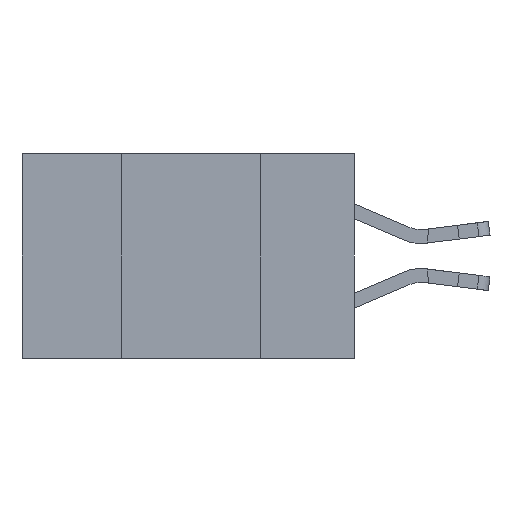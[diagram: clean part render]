
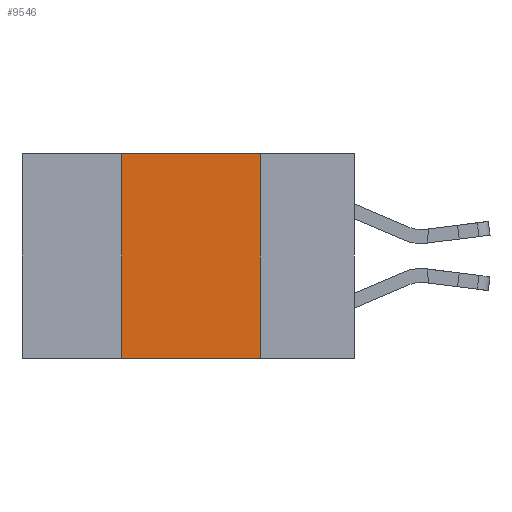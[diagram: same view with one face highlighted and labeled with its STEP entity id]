
A CAD part, left-side view. The second image highlights one B-rep face of the part: STEP entity #9546.
In plain terms, the highlighted planar face has unit normal (-1, 0, 0).
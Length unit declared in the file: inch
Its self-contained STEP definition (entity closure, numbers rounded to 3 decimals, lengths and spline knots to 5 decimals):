
#5 = ORIENTED_EDGE ( 'NONE', *, *, #11886, .F. ) ;
#1324 = CARTESIAN_POINT ( 'NONE',  ( 0., 0.6, 0. ) ) ;
#1542 = EDGE_CURVE ( 'NONE', #3734, #3479, #6570, .T. ) ;
#1946 = CARTESIAN_POINT ( 'NONE',  ( 0., 0.42, 0. ) ) ;
#2038 = VECTOR ( 'NONE', #15646, 39.37008 ) ;
#2591 = DIRECTION ( 'NONE',  ( 1., 0., 0. ) ) ;
#2919 = CARTESIAN_POINT ( 'NONE',  ( 0., 0.42, -0.37 ) ) ;
#3479 = VERTEX_POINT ( 'NONE', #3856 ) ;
#3734 = VERTEX_POINT ( 'NONE', #1946 ) ;
#3856 = CARTESIAN_POINT ( 'NONE',  ( 0., 0.17, 0. ) ) ;
#3992 = DIRECTION ( 'NONE',  ( 0., -1., 0. ) ) ;
#4912 = ORIENTED_EDGE ( 'NONE', *, *, #1542, .F. ) ;
#5870 = LINE ( 'NONE', #9533, #9399 ) ;
#6177 = VERTEX_POINT ( 'NONE', #9313 ) ;
#6570 = LINE ( 'NONE', #14681, #12372 ) ;
#6792 = ORIENTED_EDGE ( 'NONE', *, *, #10042, .T. ) ;
#8322 = DIRECTION ( 'NONE',  ( 0., 0., -1. ) ) ;
#8542 = FACE_OUTER_BOUND ( 'NONE', #12656, .T. ) ;
#8706 = PLANE ( 'NONE',  #10638 ) ;
#9276 = DIRECTION ( 'NONE',  ( 0., -1., 0. ) ) ;
#9313 = CARTESIAN_POINT ( 'NONE',  ( 0., 0.17, -0.37 ) ) ;
#9399 = VECTOR ( 'NONE', #8322, 39.37008 ) ;
#9533 = CARTESIAN_POINT ( 'NONE',  ( 0., 0.17, -0.37 ) ) ;
#9546 = ADVANCED_FACE ( 'NONE', ( #8542 ), #8706, .F. ) ;
#10027 = LINE ( 'NONE', #14874, #13368 ) ;
#10042 = EDGE_CURVE ( 'NONE', #13710, #6177, #10027, .T. ) ;
#10638 = AXIS2_PLACEMENT_3D ( 'NONE', #1324, #2591, #12453 ) ;
#10788 = LINE ( 'NONE', #10948, #2038 ) ;
#10948 = CARTESIAN_POINT ( 'NONE',  ( 0., 0.42, -0.37 ) ) ;
#11811 = EDGE_CURVE ( 'NONE', #3479, #6177, #5870, .T. ) ;
#11886 = EDGE_CURVE ( 'NONE', #13710, #3734, #10788, .T. ) ;
#12372 = VECTOR ( 'NONE', #9276, 39.37008 ) ;
#12453 = DIRECTION ( 'NONE',  ( 0., 0., -1. ) ) ;
#12656 = EDGE_LOOP ( 'NONE', ( #13865, #4912, #5, #6792 ) ) ;
#13368 = VECTOR ( 'NONE', #3992, 39.37008 ) ;
#13710 = VERTEX_POINT ( 'NONE', #2919 ) ;
#13865 = ORIENTED_EDGE ( 'NONE', *, *, #11811, .F. ) ;
#14681 = CARTESIAN_POINT ( 'NONE',  ( 0., 0.6, 0. ) ) ;
#14874 = CARTESIAN_POINT ( 'NONE',  ( 0., 0.6, -0.37 ) ) ;
#15646 = DIRECTION ( 'NONE',  ( 0., 0., 1. ) ) ;
